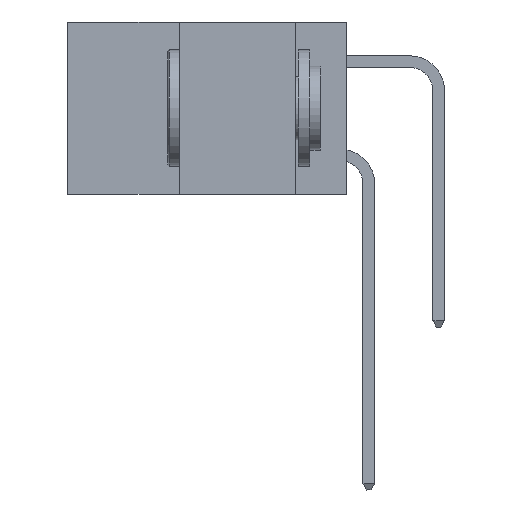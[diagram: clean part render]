
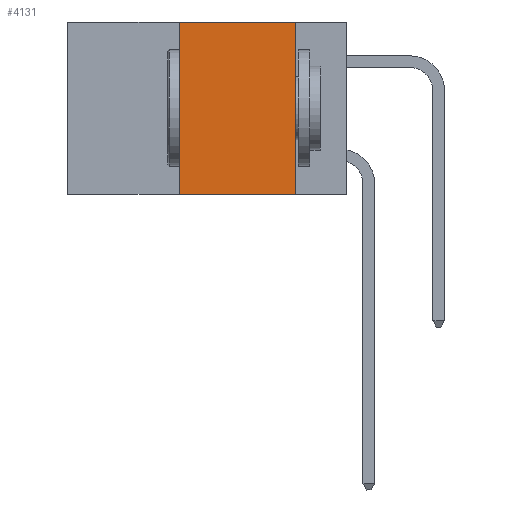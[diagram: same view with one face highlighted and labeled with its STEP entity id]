
A CAD part, left-side view. The second image highlights one B-rep face of the part: STEP entity #4131.
In plain terms, the highlighted planar face has unit normal (-1, 0, 0).
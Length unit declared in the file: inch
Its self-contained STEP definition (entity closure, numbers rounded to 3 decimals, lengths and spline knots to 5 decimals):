
#364 = VERTEX_POINT ( 'NONE', #5336 ) ;
#681 = CARTESIAN_POINT ( 'NONE',  ( 0., 0.11, 0. ) ) ;
#763 = EDGE_CURVE ( 'NONE', #4876, #364, #1991, .T. ) ;
#943 = VECTOR ( 'NONE', #3174, 39.37008 ) ;
#989 = CARTESIAN_POINT ( 'NONE',  ( 0., 0.36, 0. ) ) ;
#1042 = FACE_OUTER_BOUND ( 'NONE', #1383, .T. ) ;
#1057 = LINE ( 'NONE', #5818, #5693 ) ;
#1383 = EDGE_LOOP ( 'NONE', ( #5362, #11119, #1947, #2690 ) ) ;
#1445 = CARTESIAN_POINT ( 'NONE',  ( 0., 0.11, 0. ) ) ;
#1875 = EDGE_CURVE ( 'NONE', #8557, #3488, #8060, .T. ) ;
#1947 = ORIENTED_EDGE ( 'NONE', *, *, #1875, .F. ) ;
#1991 = LINE ( 'NONE', #681, #11734 ) ;
#2184 = DIRECTION ( 'NONE',  ( 0., -1., 0. ) ) ;
#2690 = ORIENTED_EDGE ( 'NONE', *, *, #11336, .T. ) ;
#3174 = DIRECTION ( 'NONE',  ( 0., 0., 1. ) ) ;
#3206 = VECTOR ( 'NONE', #9957, 39.37008 ) ;
#3488 = VERTEX_POINT ( 'NONE', #989 ) ;
#3620 = EDGE_CURVE ( 'NONE', #3488, #4876, #1057, .T. ) ;
#4131 = ADVANCED_FACE ( 'NONE', ( #1042 ), #10827, .F. ) ;
#4876 = VERTEX_POINT ( 'NONE', #1445 ) ;
#5336 = CARTESIAN_POINT ( 'NONE',  ( 0., 0.11, -0.37 ) ) ;
#5362 = ORIENTED_EDGE ( 'NONE', *, *, #763, .F. ) ;
#5693 = VECTOR ( 'NONE', #2184, 39.37008 ) ;
#5818 = CARTESIAN_POINT ( 'NONE',  ( 0., 0.6, 0. ) ) ;
#7157 = DIRECTION ( 'NONE',  ( 0., 0., -1. ) ) ;
#7175 = CARTESIAN_POINT ( 'NONE',  ( 0., 0.6, -0.37 ) ) ;
#8060 = LINE ( 'NONE', #11498, #943 ) ;
#8557 = VERTEX_POINT ( 'NONE', #9542 ) ;
#9542 = CARTESIAN_POINT ( 'NONE',  ( 0., 0.36, -0.37 ) ) ;
#9619 = LINE ( 'NONE', #7175, #3206 ) ;
#9932 = CARTESIAN_POINT ( 'NONE',  ( 0., 0.6, 0. ) ) ;
#9957 = DIRECTION ( 'NONE',  ( 0., -1., 0. ) ) ;
#10827 = PLANE ( 'NONE',  #11484 ) ;
#10879 = DIRECTION ( 'NONE',  ( 1., 0., 0. ) ) ;
#10983 = DIRECTION ( 'NONE',  ( 0., 0., -1. ) ) ;
#11119 = ORIENTED_EDGE ( 'NONE', *, *, #3620, .F. ) ;
#11336 = EDGE_CURVE ( 'NONE', #8557, #364, #9619, .T. ) ;
#11484 = AXIS2_PLACEMENT_3D ( 'NONE', #9932, #10879, #10983 ) ;
#11498 = CARTESIAN_POINT ( 'NONE',  ( 0., 0.36, 0. ) ) ;
#11734 = VECTOR ( 'NONE', #7157, 39.37008 ) ;
